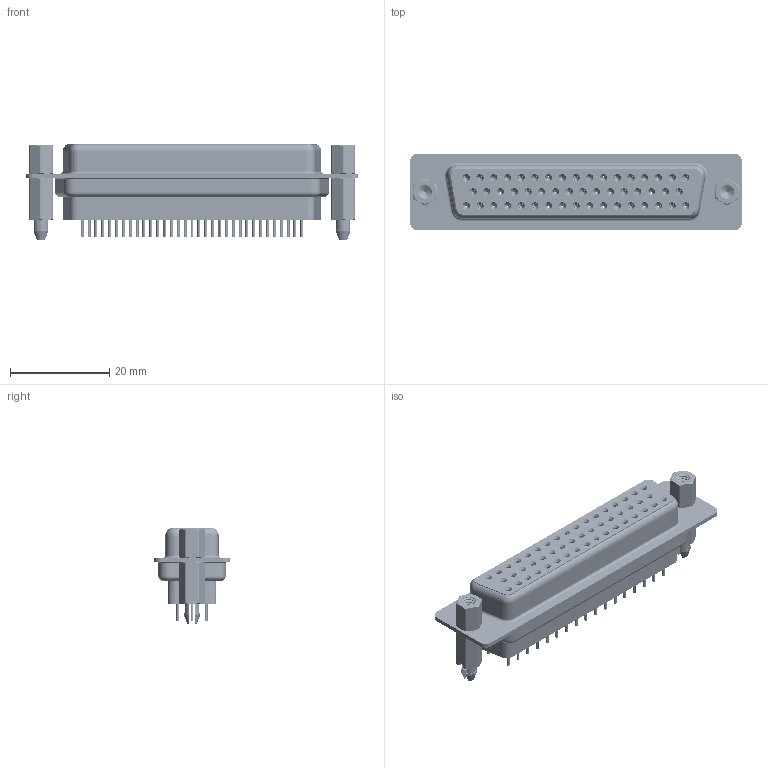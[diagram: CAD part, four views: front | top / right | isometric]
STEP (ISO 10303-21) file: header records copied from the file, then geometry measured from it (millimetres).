
FILE_DESCRIPTION (( 'STEP AP203' ), '1' );
FILE_NAME ('628-050-228-267.STEP', '2020-07-21T13:52:53', ( '' ), ( '' ), 'SwSTEP 2.0', 'SolidWorks 2020', '' );
FILE_SCHEMA (( 'CONFIG_CONTROL_DESIGN' ));
Length unit declared in the file: millimetre
Products named in the file (9): 628 Contact Row 3_28L; 628 4-40 Threaded Boardlock_FF; 628 4-40 Hex Standoff; 628 Housing_50 FF; 628-050-228-267; 628 Shell Front_50 Contacts; 628 Shell Rear_50 Contacts; 628 Contact Row 2_28L; 628 Contact Row 1_28L
Assembly tree (57 placements, depth 2):
  628-050-228-267
    628 Housing_50 FF
    628 Shell Front_50 Contacts
    628 Shell Rear_50 Contacts
    628 Contact Row 1_28L  x17
    628 Contact Row 2_28L  x16
    628 Contact Row 3_28L  x17
    628 4-40 Hex Standoff  x2
    628 4-40 Threaded Boardlock_FF  x2
Bounding box: 67 x 15.4 x 19.4 mm (x, y, z)
Volume: 8242.2 mm3; surface area: 18379.1 mm2
Topology: 58 solids, 58 shells, 7022 faces, 18032 edges, 11235 vertices
Faces by surface type: cylinder 2030, plane 1677, torus 1363, bspline 1066, cone 886
Entity records: 67318 total; most frequent: CARTESIAN_POINT 29635, DIRECTION 7678, ORIENTED_EDGE 7224, EDGE_CURVE 3612, AXIS2_PLACEMENT_3D 3211, VERTEX_POINT 2306, EDGE_LOOP 1858, CIRCLE 1760
